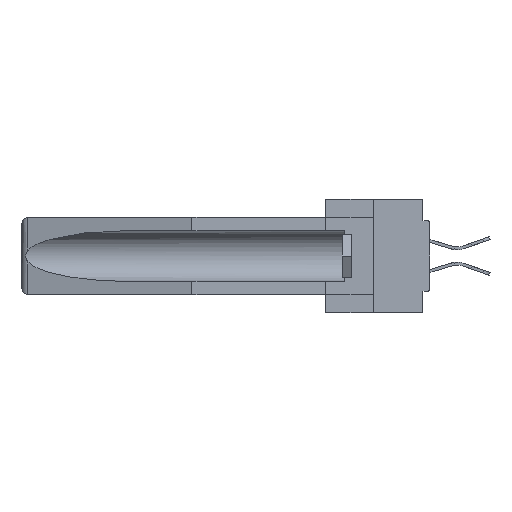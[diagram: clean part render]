
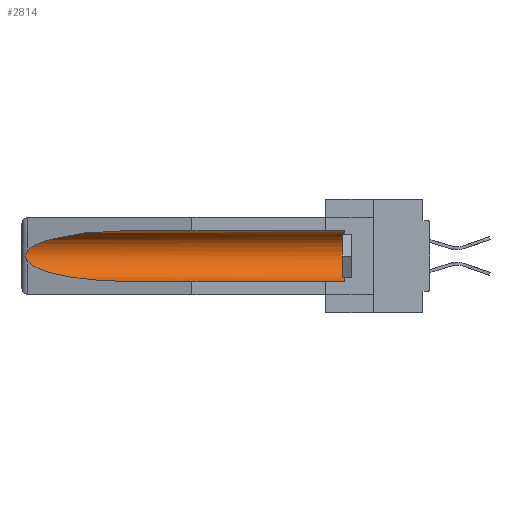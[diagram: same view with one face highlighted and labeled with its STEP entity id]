
A CAD part, left-side view. The second image highlights one B-rep face of the part: STEP entity #2814.
In plain terms, the highlighted cylindrical face has radius 2.857 mm (diameter 5.715 mm), a partial arc.
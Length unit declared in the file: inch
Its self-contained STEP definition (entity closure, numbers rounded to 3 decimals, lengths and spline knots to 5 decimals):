
#1134 = CARTESIAN_POINT ( 'NONE',  ( 0.155, 0.126, -0.284 ) ) ;
#1238 = ORIENTED_EDGE ( 'NONE', *, *, #21554, .T. ) ;
#1833 = CARTESIAN_POINT ( 'NONE',  ( 0.26537, 1.52718, -0.19328 ) ) ;
#2210 = ORIENTED_EDGE ( 'NONE', *, *, #42821, .F. ) ;
#2814 = ADVANCED_FACE ( 'NONE', ( #19639 ), #18613, .F. ) ;
#3026 = DIRECTION ( 'NONE',  ( 0., -1., 0. ) ) ;
#3355 = CARTESIAN_POINT ( 'NONE',  ( 0.21114, 1.30732, -0.059 ) ) ;
#4286 = EDGE_CURVE ( 'NONE', #28973, #32216, #25742, .T. ) ;
#4530 = ORIENTED_EDGE ( 'NONE', *, *, #43704, .T. ) ;
#5627 = VERTEX_POINT ( 'NONE', #9567 ) ;
#6736 = DIRECTION ( 'NONE',  ( 0., 1., 0. ) ) ;
#6772 = CARTESIAN_POINT ( 'NONE',  ( 0.155, 0.126, -0.1715 ) ) ;
#6805 = CARTESIAN_POINT ( 'NONE',  ( 0.25451, 1.48313, -0.09465 ) ) ;
#8472 = CARTESIAN_POINT ( 'NONE',  ( 0.2675, 1.53308, -0.17534 ) ) ;
#9478 = CARTESIAN_POINT ( 'NONE',  ( 0.155, 1.07973, -0.059 ) ) ;
#9567 = CARTESIAN_POINT ( 'NONE',  ( 0.155, 1.07973, -0.284 ) ) ;
#12022 = CARTESIAN_POINT ( 'NONE',  ( 0.26654, 1.53092, -0.15636 ) ) ;
#12026 = ORIENTED_EDGE ( 'NONE', *, *, #25653, .T. ) ;
#13246 = CARTESIAN_POINT ( 'NONE',  ( 0.155, 1.07973, -0.059 ) ) ;
#13425 = AXIS2_PLACEMENT_3D ( 'NONE', #28790, #18924, #15238 ) ;
#14139 = EDGE_CURVE ( 'NONE', #23200, #27479, #36940, .T. ) ;
#15075 = CARTESIAN_POINT ( 'NONE',  ( 0.26537, 1.52718, -0.14972 ) ) ;
#15205 = CARTESIAN_POINT ( 'NONE',  ( 0.26655, 1.53094, -0.18657 ) ) ;
#15238 = DIRECTION ( 'NONE',  ( 0., 0., 1. ) ) ;
#15568 = LINE ( 'NONE', #39577, #31996 ) ;
#17344 = VERTEX_POINT ( 'NONE', #1134 ) ;
#17376 =( BOUNDED_CURVE ( )  B_SPLINE_CURVE ( 3, ( #42496, #22001, #38829, #31911 ),
 .UNSPECIFIED., .F., .F. ) 
 B_SPLINE_CURVE_WITH_KNOTS ( ( 4, 4 ),
 ( 0.1948, 1.5708 ),
 .UNSPECIFIED. ) 
 CURVE ( )  GEOMETRIC_REPRESENTATION_ITEM ( )  RATIONAL_B_SPLINE_CURVE ( ( 1., 0.848, 0.848, 1. ) ) 
 REPRESENTATION_ITEM ( '' )  );
#17576 = AXIS2_PLACEMENT_3D ( 'NONE', #6772, #3026, #30624 ) ;
#18613 = CYLINDRICAL_SURFACE ( 'NONE', #13425, 0.1125 ) ;
#18924 = DIRECTION ( 'NONE',  ( 0., 1., 0. ) ) ;
#19639 = FACE_OUTER_BOUND ( 'NONE', #22269, .T. ) ;
#20302 = CARTESIAN_POINT ( 'NONE',  ( 0.26537, 1.52718, -0.14972 ) ) ;
#21554 = EDGE_CURVE ( 'NONE', #17344, #23200, #23085, .T. ) ;
#21563 = CARTESIAN_POINT ( 'NONE',  ( 0.26537, 1.52718, -0.19328 ) ) ;
#22001 = CARTESIAN_POINT ( 'NONE',  ( 0.25451, 1.48313, -0.24835 ) ) ;
#22269 = EDGE_LOOP ( 'NONE', ( #12026, #24423, #4530, #2210, #1238, #26348 ) ) ;
#23085 = CIRCLE ( 'NONE', #17576, 0.1125 ) ;
#23200 = VERTEX_POINT ( 'NONE', #38565 ) ;
#24423 = ORIENTED_EDGE ( 'NONE', *, *, #4286, .T. ) ;
#25216 = CARTESIAN_POINT ( 'NONE',  ( 0.26597, 1.52961, -0.15275 ) ) ;
#25653 = EDGE_CURVE ( 'NONE', #27479, #28973, #38226, .T. ) ;
#25742 = B_SPLINE_CURVE_WITH_KNOTS ( 'NONE', 3,
 ( #15075, #25216, #12022, #28334, #38669, #8472, #32335, #15205, #38395, #21563 ),
 .UNSPECIFIED., .F., .F.,
 ( 4, 2, 2, 2, 4 ),
 ( 0., 0.00029, 0.00058, 0.00087, 0.00117 ),
 .UNSPECIFIED. ) ;
#26348 = ORIENTED_EDGE ( 'NONE', *, *, #14139, .T. ) ;
#27479 = VERTEX_POINT ( 'NONE', #9478 ) ;
#28334 = CARTESIAN_POINT ( 'NONE',  ( 0.2673, 1.5327, -0.16383 ) ) ;
#28790 = CARTESIAN_POINT ( 'NONE',  ( 0.155, -0.30754, -0.1715 ) ) ;
#28973 = VERTEX_POINT ( 'NONE', #20302 ) ;
#29074 = DIRECTION ( 'NONE',  ( 0., 1., 0. ) ) ;
#30195 = CARTESIAN_POINT ( 'NONE',  ( 0.26537, 1.52718, -0.14972 ) ) ;
#30529 = CARTESIAN_POINT ( 'NONE',  ( 0.155, -0.30754, -0.059 ) ) ;
#30624 = DIRECTION ( 'NONE',  ( 0., 0., 1. ) ) ;
#31911 = CARTESIAN_POINT ( 'NONE',  ( 0.155, 1.07973, -0.284 ) ) ;
#31996 = VECTOR ( 'NONE', #6736, 39.37008 ) ;
#32216 = VERTEX_POINT ( 'NONE', #1833 ) ;
#32335 = CARTESIAN_POINT ( 'NONE',  ( 0.2673, 1.53269, -0.17917 ) ) ;
#35416 = VECTOR ( 'NONE', #29074, 39.37008 ) ;
#36940 = LINE ( 'NONE', #30529, #35416 ) ;
#38226 =( BOUNDED_CURVE ( )  B_SPLINE_CURVE ( 3, ( #13246, #3355, #6805, #30195 ),
 .UNSPECIFIED., .F., .F. ) 
 B_SPLINE_CURVE_WITH_KNOTS ( ( 4, 4 ),
 ( 4.71239, 6.08839 ),
 .UNSPECIFIED. ) 
 CURVE ( )  GEOMETRIC_REPRESENTATION_ITEM ( )  RATIONAL_B_SPLINE_CURVE ( ( 1., 0.848, 0.848, 1. ) ) 
 REPRESENTATION_ITEM ( '' )  );
#38395 = CARTESIAN_POINT ( 'NONE',  ( 0.26597, 1.5296, -0.19026 ) ) ;
#38565 = CARTESIAN_POINT ( 'NONE',  ( 0.155, 0.126, -0.059 ) ) ;
#38669 = CARTESIAN_POINT ( 'NONE',  ( 0.2675, 1.53308, -0.16763 ) ) ;
#38829 = CARTESIAN_POINT ( 'NONE',  ( 0.21114, 1.30732, -0.284 ) ) ;
#39577 = CARTESIAN_POINT ( 'NONE',  ( 0.155, -0.30754, -0.284 ) ) ;
#42496 = CARTESIAN_POINT ( 'NONE',  ( 0.26537, 1.52718, -0.19328 ) ) ;
#42821 = EDGE_CURVE ( 'NONE', #17344, #5627, #15568, .T. ) ;
#43704 = EDGE_CURVE ( 'NONE', #32216, #5627, #17376, .T. ) ;
